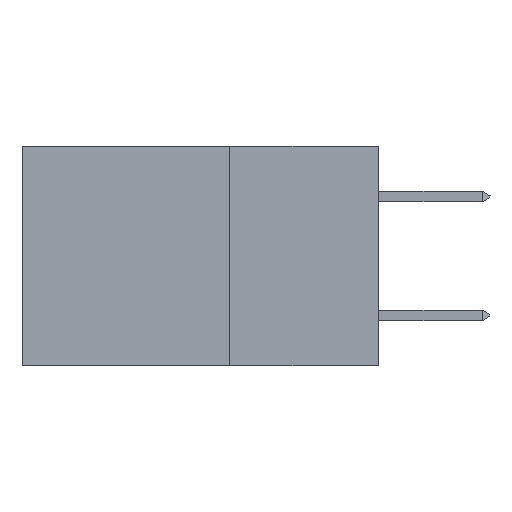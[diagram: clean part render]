
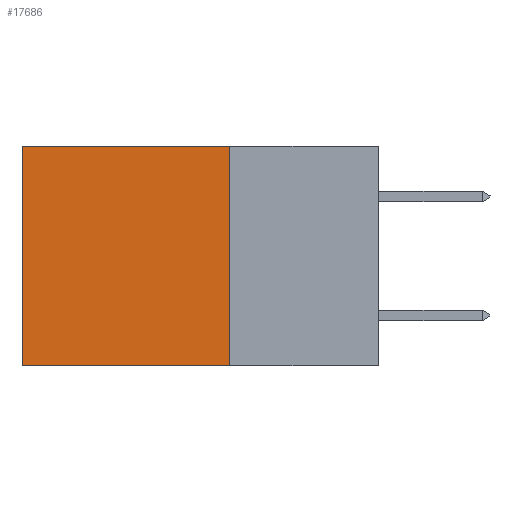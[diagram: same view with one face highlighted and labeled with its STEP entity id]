
A CAD part, left-side view. The second image highlights one B-rep face of the part: STEP entity #17686.
In plain terms, the highlighted planar face has unit normal (-1, 0, 0).
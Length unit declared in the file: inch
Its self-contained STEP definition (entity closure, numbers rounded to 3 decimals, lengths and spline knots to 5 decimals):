
#2026 = LINE ( 'NONE', #18277, #21845 ) ;
#2118 = VERTEX_POINT ( 'NONE', #19553 ) ;
#3464 = DIRECTION ( 'NONE',  ( 0., 1., 0. ) ) ;
#5285 = DIRECTION ( 'NONE',  ( 1., 0., 0. ) ) ;
#5815 = EDGE_CURVE ( 'NONE', #14080, #2118, #13227, .T. ) ;
#7610 = EDGE_CURVE ( 'NONE', #8700, #24880, #2026, .T. ) ;
#7663 = EDGE_CURVE ( 'NONE', #8700, #14080, #10088, .T. ) ;
#8118 = DIRECTION ( 'NONE',  ( 0., 0., -1. ) ) ;
#8375 = VECTOR ( 'NONE', #3464, 39.37008 ) ;
#8700 = VERTEX_POINT ( 'NONE', #10596 ) ;
#9088 = LINE ( 'NONE', #12775, #9463 ) ;
#9205 = VECTOR ( 'NONE', #8118, 39.37008 ) ;
#9463 = VECTOR ( 'NONE', #11193, 39.37008 ) ;
#10088 = LINE ( 'NONE', #16006, #9205 ) ;
#10596 = CARTESIAN_POINT ( 'NONE',  ( 0.2615, 0.25, 0. ) ) ;
#11193 = DIRECTION ( 'NONE',  ( 0., 0., -1. ) ) ;
#11210 = ORIENTED_EDGE ( 'NONE', *, *, #7610, .T. ) ;
#12775 = CARTESIAN_POINT ( 'NONE',  ( 0.2615, 0.6, -0.37 ) ) ;
#13227 = LINE ( 'NONE', #23681, #8375 ) ;
#13315 = DIRECTION ( 'NONE',  ( 0., 0., -1. ) ) ;
#13887 = DIRECTION ( 'NONE',  ( 0., 1., 0. ) ) ;
#14080 = VERTEX_POINT ( 'NONE', #14879 ) ;
#14875 = ORIENTED_EDGE ( 'NONE', *, *, #7663, .F. ) ;
#14879 = CARTESIAN_POINT ( 'NONE',  ( 0.2615, 0.25, -0.37 ) ) ;
#15932 = ORIENTED_EDGE ( 'NONE', *, *, #18020, .T. ) ;
#16006 = CARTESIAN_POINT ( 'NONE',  ( 0.2615, 0.25, -0.37 ) ) ;
#16801 = CARTESIAN_POINT ( 'NONE',  ( 0.2615, 0.6, 0. ) ) ;
#17018 = AXIS2_PLACEMENT_3D ( 'NONE', #21001, #5285, #13315 ) ;
#17686 = ADVANCED_FACE ( 'NONE', ( #25399 ), #22870, .F. ) ;
#18012 = EDGE_LOOP ( 'NONE', ( #15932, #24403, #14875, #11210 ) ) ;
#18020 = EDGE_CURVE ( 'NONE', #24880, #2118, #9088, .T. ) ;
#18277 = CARTESIAN_POINT ( 'NONE',  ( 0.2615, 0.25, 0. ) ) ;
#19553 = CARTESIAN_POINT ( 'NONE',  ( 0.2615, 0.6, -0.37 ) ) ;
#21001 = CARTESIAN_POINT ( 'NONE',  ( 0.2615, 0.25, -0.37 ) ) ;
#21845 = VECTOR ( 'NONE', #13887, 39.37008 ) ;
#22870 = PLANE ( 'NONE',  #17018 ) ;
#23681 = CARTESIAN_POINT ( 'NONE',  ( 0.2615, 0.25, -0.37 ) ) ;
#24403 = ORIENTED_EDGE ( 'NONE', *, *, #5815, .F. ) ;
#24880 = VERTEX_POINT ( 'NONE', #16801 ) ;
#25399 = FACE_OUTER_BOUND ( 'NONE', #18012, .T. ) ;
